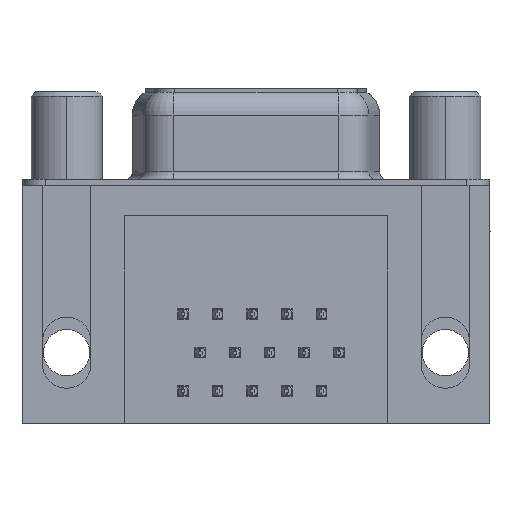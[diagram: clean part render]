
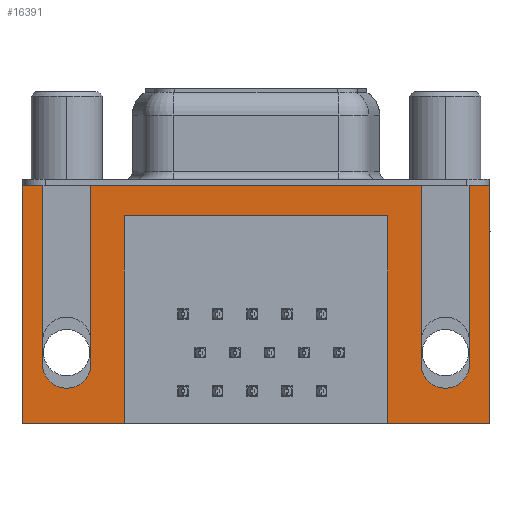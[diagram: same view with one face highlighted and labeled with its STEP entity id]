
A CAD part, front view. The second image highlights one B-rep face of the part: STEP entity #16391.
In plain terms, the highlighted planar face has unit normal (0, -1, 0).
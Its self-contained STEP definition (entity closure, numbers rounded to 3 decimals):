
#191 = EDGE_CURVE ( 'NONE', #24638, #25841, #11512, .T. ) ;
#216 = CARTESIAN_POINT ( 'NONE',  ( 27.9, -6.275, 0. ) ) ;
#624 = CARTESIAN_POINT ( 'NONE',  ( 3.79, -6.275, -2. ) ) ;
#632 = LINE ( 'NONE', #23113, #28561 ) ;
#891 = CARTESIAN_POINT ( 'NONE',  ( -2.91, -6.275, 0. ) ) ;
#1148 = DIRECTION ( 'NONE',  ( 0., 0., 1. ) ) ;
#2147 = CARTESIAN_POINT ( 'NONE',  ( 26.59, -6.275, 0. ) ) ;
#2192 = DIRECTION ( 'NONE',  ( 0., 0., 1. ) ) ;
#2213 = VECTOR ( 'NONE', #10977, 1000. ) ;
#2316 = LINE ( 'NONE', #32503, #9969 ) ;
#2844 = ORIENTED_EDGE ( 'NONE', *, *, #16320, .F. ) ;
#3298 = CARTESIAN_POINT ( 'NONE',  ( -1.6, -6.275, 0. ) ) ;
#3348 = CARTESIAN_POINT ( 'NONE',  ( 23.39, -6.275, 0. ) ) ;
#4180 = CARTESIAN_POINT ( 'NONE',  ( -2.91, -6.275, -2.5 ) ) ;
#4290 = EDGE_CURVE ( 'NONE', #14889, #24206, #16754, .T. ) ;
#4812 = ORIENTED_EDGE ( 'NONE', *, *, #6864, .F. ) ;
#5064 = EDGE_CURVE ( 'NONE', #7073, #18703, #2316, .T. ) ;
#5106 = CARTESIAN_POINT ( 'NONE',  ( -2.91, -6.275, -15.7 ) ) ;
#5107 = ORIENTED_EDGE ( 'NONE', *, *, #13922, .F. ) ;
#5335 = DIRECTION ( 'NONE',  ( -1., 0., 0. ) ) ;
#5582 = VERTEX_POINT ( 'NONE', #29095 ) ;
#5616 = EDGE_CURVE ( 'NONE', #25286, #7073, #18475, .T. ) ;
#5687 = CIRCLE ( 'NONE', #33348, 1.6 ) ;
#5722 = DIRECTION ( 'NONE',  ( 0., 0., 1. ) ) ;
#5868 = LINE ( 'NONE', #36694, #27921 ) ;
#6864 = EDGE_CURVE ( 'NONE', #24384, #24638, #9875, .T. ) ;
#7073 = VERTEX_POINT ( 'NONE', #35043 ) ;
#7102 = DIRECTION ( 'NONE',  ( 0., 0., -1. ) ) ;
#7256 = LINE ( 'NONE', #2147, #13979 ) ;
#7664 = VERTEX_POINT ( 'NONE', #8523 ) ;
#7684 = VERTEX_POINT ( 'NONE', #216 ) ;
#8523 = CARTESIAN_POINT ( 'NONE',  ( -1.6, -6.275, -11.78 ) ) ;
#8751 = DIRECTION ( 'NONE',  ( 0., 0., -1. ) ) ;
#8885 = DIRECTION ( 'NONE',  ( 1., 0., 0. ) ) ;
#9408 = CARTESIAN_POINT ( 'NONE',  ( 26.59, -6.275, -11.78 ) ) ;
#9798 = EDGE_LOOP ( 'NONE', ( #24877, #28168, #2844, #14176, #4812, #12040, #33982, #20451, #25481, #23405, #36376, #15765, #28661, #14941, #37187, #5107 ) ) ;
#9875 = LINE ( 'NONE', #25294, #2213 ) ;
#9969 = VECTOR ( 'NONE', #5335, 1000. ) ;
#9973 = EDGE_CURVE ( 'NONE', #7664, #24384, #5687, .T. ) ;
#10304 = DIRECTION ( 'NONE',  ( 1., 0., 0. ) ) ;
#10789 = CARTESIAN_POINT ( 'NONE',  ( 1.6, -6.275, -11.78 ) ) ;
#10819 = VECTOR ( 'NONE', #26547, 1000. ) ;
#10977 = DIRECTION ( 'NONE',  ( 0., 0., 1. ) ) ;
#11464 = LINE ( 'NONE', #11658, #33614 ) ;
#11512 = LINE ( 'NONE', #35575, #26840 ) ;
#11648 = EDGE_CURVE ( 'NONE', #24206, #7664, #11464, .T. ) ;
#11658 = CARTESIAN_POINT ( 'NONE',  ( -1.6, -6.275, 0. ) ) ;
#12040 = ORIENTED_EDGE ( 'NONE', *, *, #9973, .F. ) ;
#12301 = DIRECTION ( 'NONE',  ( 1., 0., 0. ) ) ;
#12579 = CARTESIAN_POINT ( 'NONE',  ( -2.91, -6.275, -2.5 ) ) ;
#12599 = DIRECTION ( 'NONE',  ( 0., 0., -1. ) ) ;
#13042 = CARTESIAN_POINT ( 'NONE',  ( 21.2, -6.275, -2. ) ) ;
#13043 = AXIS2_PLACEMENT_3D ( 'NONE', #4180, #24307, #7102 ) ;
#13922 = EDGE_CURVE ( 'NONE', #30963, #7684, #32105, .T. ) ;
#13947 = LINE ( 'NONE', #20036, #35167 ) ;
#13979 = VECTOR ( 'NONE', #33882, 1000. ) ;
#14176 = ORIENTED_EDGE ( 'NONE', *, *, #191, .F. ) ;
#14781 = CARTESIAN_POINT ( 'NONE',  ( 26.59, -6.275, 0. ) ) ;
#14889 = VERTEX_POINT ( 'NONE', #891 ) ;
#14941 = ORIENTED_EDGE ( 'NONE', *, *, #20291, .F. ) ;
#15223 = EDGE_CURVE ( 'NONE', #19861, #30963, #7256, .T. ) ;
#15431 = VERTEX_POINT ( 'NONE', #20571 ) ;
#15670 = DIRECTION ( 'NONE',  ( 0., -1., 0. ) ) ;
#15765 = ORIENTED_EDGE ( 'NONE', *, *, #32376, .F. ) ;
#16023 = EDGE_CURVE ( 'NONE', #15431, #23153, #13947, .T. ) ;
#16191 = DIRECTION ( 'NONE',  ( 0., -1., 0. ) ) ;
#16250 = CARTESIAN_POINT ( 'NONE',  ( 3.79, -6.275, -2. ) ) ;
#16320 = EDGE_CURVE ( 'NONE', #25841, #37364, #32809, .T. ) ;
#16391 = ADVANCED_FACE ( 'NONE', ( #24716 ), #18528, .T. ) ;
#16548 = LINE ( 'NONE', #12579, #30987 ) ;
#16754 = LINE ( 'NONE', #34380, #32074 ) ;
#17893 = EDGE_CURVE ( 'NONE', #18703, #14889, #16548, .T. ) ;
#18475 = LINE ( 'NONE', #624, #10819 ) ;
#18528 = PLANE ( 'NONE',  #13043 ) ;
#18703 = VERTEX_POINT ( 'NONE', #5106 ) ;
#19391 = CARTESIAN_POINT ( 'NONE',  ( -2.91, -6.275, 0. ) ) ;
#19861 = VERTEX_POINT ( 'NONE', #9408 ) ;
#20036 = CARTESIAN_POINT ( 'NONE',  ( 21.2, -6.275, -2. ) ) ;
#20094 = VECTOR ( 'NONE', #30745, 1000. ) ;
#20291 = EDGE_CURVE ( 'NONE', #5582, #15431, #632, .T. ) ;
#20451 = ORIENTED_EDGE ( 'NONE', *, *, #4290, .F. ) ;
#20571 = CARTESIAN_POINT ( 'NONE',  ( 21.2, -6.275, -15.7 ) ) ;
#21007 = LINE ( 'NONE', #16250, #20094 ) ;
#23113 = CARTESIAN_POINT ( 'NONE',  ( 27.9, -6.275, -15.7 ) ) ;
#23153 = VERTEX_POINT ( 'NONE', #13042 ) ;
#23405 = ORIENTED_EDGE ( 'NONE', *, *, #5064, .F. ) ;
#24206 = VERTEX_POINT ( 'NONE', #3298 ) ;
#24307 = DIRECTION ( 'NONE',  ( 0., -1., 0. ) ) ;
#24384 = VERTEX_POINT ( 'NONE', #10789 ) ;
#24638 = VERTEX_POINT ( 'NONE', #29288 ) ;
#24716 = FACE_OUTER_BOUND ( 'NONE', #9798, .T. ) ;
#24877 = ORIENTED_EDGE ( 'NONE', *, *, #15223, .F. ) ;
#25286 = VERTEX_POINT ( 'NONE', #33009 ) ;
#25294 = CARTESIAN_POINT ( 'NONE',  ( 1.6, -6.275, 0. ) ) ;
#25481 = ORIENTED_EDGE ( 'NONE', *, *, #17893, .F. ) ;
#25604 = VECTOR ( 'NONE', #12599, 1000. ) ;
#25841 = VERTEX_POINT ( 'NONE', #3348 ) ;
#26054 = EDGE_CURVE ( 'NONE', #37364, #19861, #33928, .T. ) ;
#26547 = DIRECTION ( 'NONE',  ( 0., 0., -1. ) ) ;
#26840 = VECTOR ( 'NONE', #10304, 1000. ) ;
#27921 = VECTOR ( 'NONE', #2192, 1000. ) ;
#28067 = DIRECTION ( 'NONE',  ( 1., 0., 0. ) ) ;
#28168 = ORIENTED_EDGE ( 'NONE', *, *, #26054, .F. ) ;
#28561 = VECTOR ( 'NONE', #34647, 1000. ) ;
#28661 = ORIENTED_EDGE ( 'NONE', *, *, #16023, .F. ) ;
#29095 = CARTESIAN_POINT ( 'NONE',  ( 27.9, -6.275, -15.7 ) ) ;
#29288 = CARTESIAN_POINT ( 'NONE',  ( 1.6, -6.275, 0. ) ) ;
#30067 = EDGE_CURVE ( 'NONE', #5582, #7684, #5868, .T. ) ;
#30410 = CARTESIAN_POINT ( 'NONE',  ( 0., -6.275, -11.78 ) ) ;
#30745 = DIRECTION ( 'NONE',  ( -1., 0., 0. ) ) ;
#30963 = VERTEX_POINT ( 'NONE', #14781 ) ;
#30987 = VECTOR ( 'NONE', #1148, 1000. ) ;
#31208 = VECTOR ( 'NONE', #28067, 1000. ) ;
#32074 = VECTOR ( 'NONE', #8885, 1000. ) ;
#32105 = LINE ( 'NONE', #19391, #31208 ) ;
#32376 = EDGE_CURVE ( 'NONE', #23153, #25286, #21007, .T. ) ;
#32503 = CARTESIAN_POINT ( 'NONE',  ( 27.9, -6.275, -15.7 ) ) ;
#32809 = LINE ( 'NONE', #35572, #25604 ) ;
#33009 = CARTESIAN_POINT ( 'NONE',  ( 3.79, -6.275, -2. ) ) ;
#33348 = AXIS2_PLACEMENT_3D ( 'NONE', #30410, #15670, #12301 ) ;
#33470 = CARTESIAN_POINT ( 'NONE',  ( 24.99, -6.275, -11.78 ) ) ;
#33614 = VECTOR ( 'NONE', #8751, 1000. ) ;
#33882 = DIRECTION ( 'NONE',  ( 0., 0., 1. ) ) ;
#33928 = CIRCLE ( 'NONE', #35345, 1.6 ) ;
#33982 = ORIENTED_EDGE ( 'NONE', *, *, #11648, .F. ) ;
#34380 = CARTESIAN_POINT ( 'NONE',  ( -2.91, -6.275, 0. ) ) ;
#34647 = DIRECTION ( 'NONE',  ( -1., 0., 0. ) ) ;
#35043 = CARTESIAN_POINT ( 'NONE',  ( 3.79, -6.275, -15.7 ) ) ;
#35167 = VECTOR ( 'NONE', #5722, 1000. ) ;
#35345 = AXIS2_PLACEMENT_3D ( 'NONE', #33470, #16191, #36368 ) ;
#35572 = CARTESIAN_POINT ( 'NONE',  ( 23.39, -6.275, 0. ) ) ;
#35575 = CARTESIAN_POINT ( 'NONE',  ( -2.91, -6.275, 0. ) ) ;
#35606 = CARTESIAN_POINT ( 'NONE',  ( 23.39, -6.275, -11.78 ) ) ;
#36368 = DIRECTION ( 'NONE',  ( -1., 0., 0. ) ) ;
#36376 = ORIENTED_EDGE ( 'NONE', *, *, #5616, .F. ) ;
#36694 = CARTESIAN_POINT ( 'NONE',  ( 27.9, -6.275, -2.5 ) ) ;
#37187 = ORIENTED_EDGE ( 'NONE', *, *, #30067, .T. ) ;
#37364 = VERTEX_POINT ( 'NONE', #35606 ) ;
